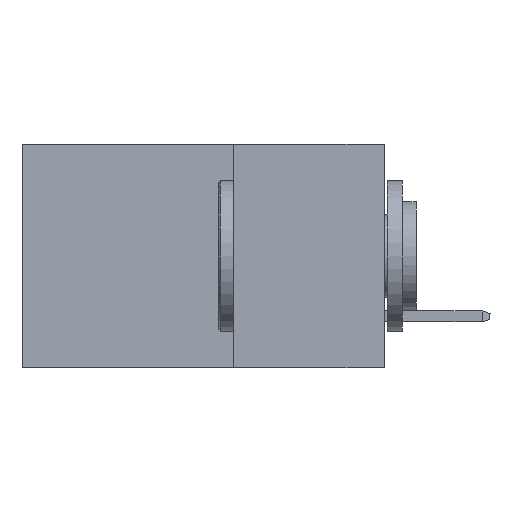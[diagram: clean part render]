
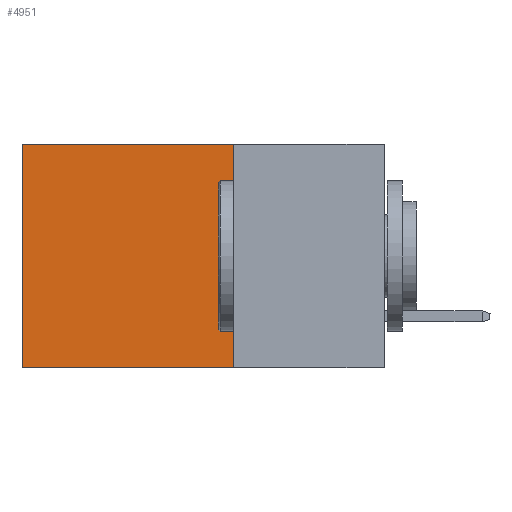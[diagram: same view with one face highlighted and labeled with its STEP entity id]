
A CAD part, left-side view. The second image highlights one B-rep face of the part: STEP entity #4951.
In plain terms, the highlighted planar face has unit normal (-1, 0, 0).
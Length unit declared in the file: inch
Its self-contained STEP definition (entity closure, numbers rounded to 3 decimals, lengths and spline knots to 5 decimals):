
#758 = CARTESIAN_POINT ( 'NONE',  ( 0.2615, 0.6, -0.37 ) ) ;
#854 = CARTESIAN_POINT ( 'NONE',  ( 0.2615, 0.25, -0.37 ) ) ;
#856 = LINE ( 'NONE', #758, #19693 ) ;
#1699 = CARTESIAN_POINT ( 'NONE',  ( 0.2615, 0.25, 0. ) ) ;
#1717 = VERTEX_POINT ( 'NONE', #19019 ) ;
#2324 = LINE ( 'NONE', #3828, #19436 ) ;
#2358 = DIRECTION ( 'NONE',  ( 0., 0., -1. ) ) ;
#3202 = ORIENTED_EDGE ( 'NONE', *, *, #20379, .F. ) ;
#3276 = CARTESIAN_POINT ( 'NONE',  ( 0.2615, 0.6, 0. ) ) ;
#3355 = VECTOR ( 'NONE', #6835, 39.37008 ) ;
#3828 = CARTESIAN_POINT ( 'NONE',  ( 0.2615, 0.25, -0.37 ) ) ;
#4951 = ADVANCED_FACE ( 'NONE', ( #20519 ), #12299, .F. ) ;
#5572 = ORIENTED_EDGE ( 'NONE', *, *, #15933, .T. ) ;
#5776 = VERTEX_POINT ( 'NONE', #10423 ) ;
#6835 = DIRECTION ( 'NONE',  ( 0., 0., -1. ) ) ;
#7262 = ORIENTED_EDGE ( 'NONE', *, *, #15760, .T. ) ;
#7690 = DIRECTION ( 'NONE',  ( 0., 0., -1. ) ) ;
#10423 = CARTESIAN_POINT ( 'NONE',  ( 0.2615, 0.25, 0. ) ) ;
#11808 = VERTEX_POINT ( 'NONE', #3276 ) ;
#12299 = PLANE ( 'NONE',  #12838 ) ;
#12838 = AXIS2_PLACEMENT_3D ( 'NONE', #854, #15600, #7690 ) ;
#13339 = LINE ( 'NONE', #1699, #15974 ) ;
#14955 = ORIENTED_EDGE ( 'NONE', *, *, #17394, .F. ) ;
#15470 = DIRECTION ( 'NONE',  ( 0., 1., 0. ) ) ;
#15600 = DIRECTION ( 'NONE',  ( 1., 0., 0. ) ) ;
#15760 = EDGE_CURVE ( 'NONE', #11808, #1717, #856, .T. ) ;
#15933 = EDGE_CURVE ( 'NONE', #5776, #11808, #13339, .T. ) ;
#15974 = VECTOR ( 'NONE', #16343, 39.37008 ) ;
#16343 = DIRECTION ( 'NONE',  ( 0., 1., 0. ) ) ;
#16810 = VERTEX_POINT ( 'NONE', #19248 ) ;
#17394 = EDGE_CURVE ( 'NONE', #5776, #16810, #18038, .T. ) ;
#18019 = EDGE_LOOP ( 'NONE', ( #7262, #3202, #14955, #5572 ) ) ;
#18038 = LINE ( 'NONE', #19764, #3355 ) ;
#19019 = CARTESIAN_POINT ( 'NONE',  ( 0.2615, 0.6, -0.37 ) ) ;
#19248 = CARTESIAN_POINT ( 'NONE',  ( 0.2615, 0.25, -0.37 ) ) ;
#19436 = VECTOR ( 'NONE', #15470, 39.37008 ) ;
#19693 = VECTOR ( 'NONE', #2358, 39.37008 ) ;
#19764 = CARTESIAN_POINT ( 'NONE',  ( 0.2615, 0.25, -0.37 ) ) ;
#20379 = EDGE_CURVE ( 'NONE', #16810, #1717, #2324, .T. ) ;
#20519 = FACE_OUTER_BOUND ( 'NONE', #18019, .T. ) ;
